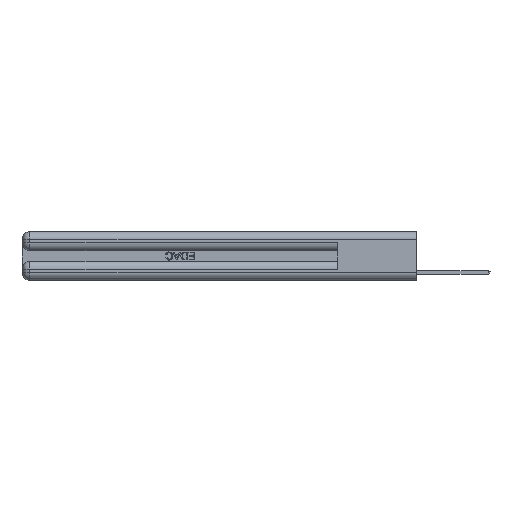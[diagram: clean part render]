
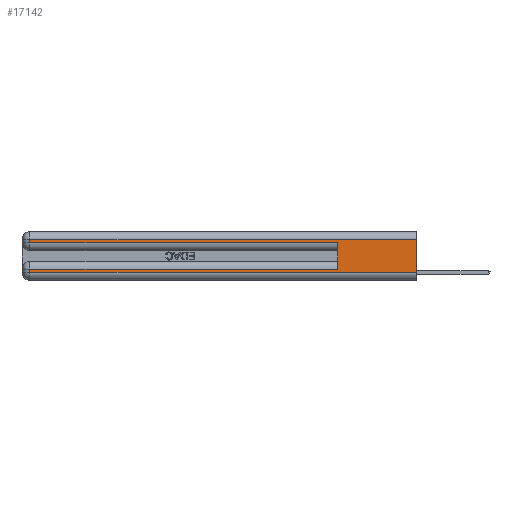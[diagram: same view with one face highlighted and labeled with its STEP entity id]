
A CAD part, left-side view. The second image highlights one B-rep face of the part: STEP entity #17142.
In plain terms, the highlighted planar face has unit normal (-1, 0, 0).
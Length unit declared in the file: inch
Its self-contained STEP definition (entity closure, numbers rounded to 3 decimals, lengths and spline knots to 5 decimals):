
#565 = VERTEX_POINT ( 'NONE', #15752 ) ;
#574 = DIRECTION ( 'NONE',  ( 0., 0., -1. ) ) ;
#761 = AXIS2_PLACEMENT_3D ( 'NONE', #23906, #26320, #15889 ) ;
#1236 = EDGE_CURVE ( 'NONE', #565, #13923, #27233, .T. ) ;
#1604 = CARTESIAN_POINT ( 'NONE',  ( 0., 0., 0.085 ) ) ;
#2051 = CARTESIAN_POINT ( 'NONE',  ( 0., 0., 0.31 ) ) ;
#2996 = CARTESIAN_POINT ( 'NONE',  ( 0., 2.94, 0.31 ) ) ;
#3161 = EDGE_CURVE ( 'NONE', #18981, #27182, #19960, .T. ) ;
#3506 = VECTOR ( 'NONE', #22042, 39.37008 ) ;
#4141 = LINE ( 'NONE', #2051, #7210 ) ;
#4173 = LINE ( 'NONE', #1604, #8993 ) ;
#4622 = DIRECTION ( 'NONE',  ( 0., 0., 1. ) ) ;
#4841 = CARTESIAN_POINT ( 'NONE',  ( 0., 2.94, 0.285 ) ) ;
#5101 = VERTEX_POINT ( 'NONE', #4841 ) ;
#5821 = DIRECTION ( 'NONE',  ( 0., -1., 0. ) ) ;
#6107 = EDGE_CURVE ( 'NONE', #13923, #27182, #10932, .T. ) ;
#6274 = FACE_OUTER_BOUND ( 'NONE', #12779, .T. ) ;
#6540 = CARTESIAN_POINT ( 'NONE',  ( 0., 0.6, 0.085 ) ) ;
#6697 = CARTESIAN_POINT ( 'NONE',  ( 0., 2.94, 0.06 ) ) ;
#6873 = DIRECTION ( 'NONE',  ( 0., 1., 0. ) ) ;
#7194 = DIRECTION ( 'NONE',  ( 0., 0., -1. ) ) ;
#7210 = VECTOR ( 'NONE', #6873, 39.37008 ) ;
#7688 = EDGE_CURVE ( 'NONE', #25803, #5101, #9698, .T. ) ;
#8084 = LINE ( 'NONE', #27654, #21431 ) ;
#8993 = VECTOR ( 'NONE', #20990, 39.37008 ) ;
#9698 = LINE ( 'NONE', #19471, #3506 ) ;
#9953 = ORIENTED_EDGE ( 'NONE', *, *, #7688, .T. ) ;
#10932 = LINE ( 'NONE', #11247, #17345 ) ;
#11247 = CARTESIAN_POINT ( 'NONE',  ( 0., 0., 0.06 ) ) ;
#11281 = VECTOR ( 'NONE', #4622, 39.37008 ) ;
#12779 = EDGE_LOOP ( 'NONE', ( #24373, #20049, #9953, #30300, #31539, #13442, #23927, #26071 ) ) ;
#13442 = ORIENTED_EDGE ( 'NONE', *, *, #21167, .T. ) ;
#13450 = CARTESIAN_POINT ( 'NONE',  ( 0., 0.6, 0.285 ) ) ;
#13923 = VERTEX_POINT ( 'NONE', #6697 ) ;
#15752 = CARTESIAN_POINT ( 'NONE',  ( 0., 2.94, 0.085 ) ) ;
#15889 = DIRECTION ( 'NONE',  ( 0., 0., -1. ) ) ;
#16537 = PLANE ( 'NONE',  #761 ) ;
#17142 = ADVANCED_FACE ( 'NONE', ( #6274 ), #16537, .F. ) ;
#17345 = VECTOR ( 'NONE', #5821, 39.37008 ) ;
#17717 = CARTESIAN_POINT ( 'NONE',  ( 0., 0., 0.37 ) ) ;
#18981 = VERTEX_POINT ( 'NONE', #29643 ) ;
#19203 = CARTESIAN_POINT ( 'NONE',  ( 0., 0.6, 0.145 ) ) ;
#19471 = CARTESIAN_POINT ( 'NONE',  ( 0., 2.94, 0.37 ) ) ;
#19960 = LINE ( 'NONE', #17717, #23486 ) ;
#20049 = ORIENTED_EDGE ( 'NONE', *, *, #28254, .T. ) ;
#20413 = DIRECTION ( 'NONE',  ( 0., -1., 0. ) ) ;
#20933 = CARTESIAN_POINT ( 'NONE',  ( 0., 0., 0.06 ) ) ;
#20990 = DIRECTION ( 'NONE',  ( 0., 1., 0. ) ) ;
#21167 = EDGE_CURVE ( 'NONE', #24174, #565, #4173, .T. ) ;
#21431 = VECTOR ( 'NONE', #20413, 39.37008 ) ;
#22042 = DIRECTION ( 'NONE',  ( 0., 0., -1. ) ) ;
#23486 = VECTOR ( 'NONE', #574, 39.37008 ) ;
#23703 = LINE ( 'NONE', #19203, #11281 ) ;
#23906 = CARTESIAN_POINT ( 'NONE',  ( 0., 0., 0.37 ) ) ;
#23927 = ORIENTED_EDGE ( 'NONE', *, *, #1236, .T. ) ;
#24174 = VERTEX_POINT ( 'NONE', #6540 ) ;
#24373 = ORIENTED_EDGE ( 'NONE', *, *, #3161, .F. ) ;
#25803 = VERTEX_POINT ( 'NONE', #2996 ) ;
#26071 = ORIENTED_EDGE ( 'NONE', *, *, #6107, .T. ) ;
#26320 = DIRECTION ( 'NONE',  ( 1., 0., 0. ) ) ;
#26385 = EDGE_CURVE ( 'NONE', #5101, #28814, #8084, .T. ) ;
#27070 = CARTESIAN_POINT ( 'NONE',  ( 0., 2.94, 0.37 ) ) ;
#27182 = VERTEX_POINT ( 'NONE', #20933 ) ;
#27233 = LINE ( 'NONE', #27070, #28059 ) ;
#27654 = CARTESIAN_POINT ( 'NONE',  ( 0., 0., 0.285 ) ) ;
#28059 = VECTOR ( 'NONE', #7194, 39.37008 ) ;
#28254 = EDGE_CURVE ( 'NONE', #18981, #25803, #4141, .T. ) ;
#28333 = EDGE_CURVE ( 'NONE', #24174, #28814, #23703, .T. ) ;
#28814 = VERTEX_POINT ( 'NONE', #13450 ) ;
#29643 = CARTESIAN_POINT ( 'NONE',  ( 0., 0., 0.31 ) ) ;
#30300 = ORIENTED_EDGE ( 'NONE', *, *, #26385, .T. ) ;
#31539 = ORIENTED_EDGE ( 'NONE', *, *, #28333, .F. ) ;
